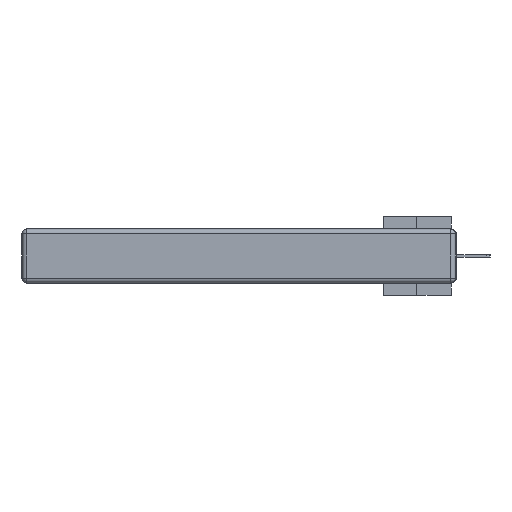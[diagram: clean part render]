
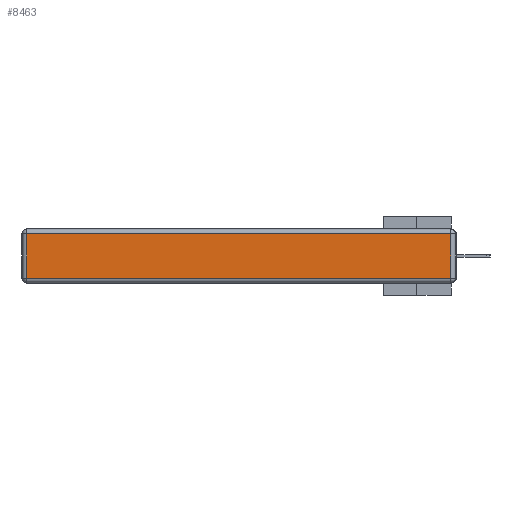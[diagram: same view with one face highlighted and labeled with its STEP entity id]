
A CAD part, left-side view. The second image highlights one B-rep face of the part: STEP entity #8463.
In plain terms, the highlighted planar face has unit normal (-1, 0, 0).
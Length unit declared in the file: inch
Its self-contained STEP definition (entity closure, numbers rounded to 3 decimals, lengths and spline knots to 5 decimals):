
#387 = VERTEX_POINT ( 'NONE', #8838 ) ;
#856 = VERTEX_POINT ( 'NONE', #28728 ) ;
#1134 = DIRECTION ( 'NONE',  ( 0., 0., -1. ) ) ;
#1557 = EDGE_CURVE ( 'NONE', #30566, #7993, #21441, .T. ) ;
#2081 = EDGE_CURVE ( 'NONE', #856, #387, #15373, .T. ) ;
#2544 = DIRECTION ( 'NONE',  ( -1., 0., 0. ) ) ;
#3279 = ORIENTED_EDGE ( 'NONE', *, *, #2081, .T. ) ;
#3412 = VECTOR ( 'NONE', #26601, 39.37008 ) ;
#4105 = EDGE_LOOP ( 'NONE', ( #13180, #20507, #6673, #3279 ) ) ;
#4881 = CARTESIAN_POINT ( 'NONE',  ( 0., 0., -0.343 ) ) ;
#6668 = VECTOR ( 'NONE', #13148, 39.37008 ) ;
#6673 = ORIENTED_EDGE ( 'NONE', *, *, #18201, .T. ) ;
#7993 = VERTEX_POINT ( 'NONE', #28312 ) ;
#8420 = CARTESIAN_POINT ( 'NONE',  ( 0., 2.72, -0.343 ) ) ;
#8463 = ADVANCED_FACE ( 'NONE', ( #26084 ), #23743, .T. ) ;
#8838 = CARTESIAN_POINT ( 'NONE',  ( 0., 2.72, -0.313 ) ) ;
#9593 = CARTESIAN_POINT ( 'NONE',  ( 0., 2.75, -0.03 ) ) ;
#11919 = DIRECTION ( 'NONE',  ( 0., 1., 0. ) ) ;
#11995 = DIRECTION ( 'NONE',  ( 0., 0., 1. ) ) ;
#13148 = DIRECTION ( 'NONE',  ( 0., -1., 0. ) ) ;
#13180 = ORIENTED_EDGE ( 'NONE', *, *, #23139, .T. ) ;
#14557 = AXIS2_PLACEMENT_3D ( 'NONE', #4881, #2544, #11995 ) ;
#15373 = LINE ( 'NONE', #8420, #22753 ) ;
#18201 = EDGE_CURVE ( 'NONE', #7993, #856, #23813, .T. ) ;
#18370 = CARTESIAN_POINT ( 'NONE',  ( 0., 0., -0.313 ) ) ;
#20266 = VECTOR ( 'NONE', #11919, 39.37008 ) ;
#20478 = CARTESIAN_POINT ( 'NONE',  ( 0., 0.03, -0.313 ) ) ;
#20507 = ORIENTED_EDGE ( 'NONE', *, *, #1557, .T. ) ;
#21441 = LINE ( 'NONE', #21593, #3412 ) ;
#21593 = CARTESIAN_POINT ( 'NONE',  ( 0., 0.03, -0.343 ) ) ;
#22753 = VECTOR ( 'NONE', #1134, 39.37008 ) ;
#23139 = EDGE_CURVE ( 'NONE', #387, #30566, #27885, .T. ) ;
#23743 = PLANE ( 'NONE',  #14557 ) ;
#23813 = LINE ( 'NONE', #9593, #20266 ) ;
#26084 = FACE_OUTER_BOUND ( 'NONE', #4105, .T. ) ;
#26601 = DIRECTION ( 'NONE',  ( 0., 0., 1. ) ) ;
#27885 = LINE ( 'NONE', #18370, #6668 ) ;
#28312 = CARTESIAN_POINT ( 'NONE',  ( 0., 0.03, -0.03 ) ) ;
#28728 = CARTESIAN_POINT ( 'NONE',  ( 0., 2.72, -0.03 ) ) ;
#30566 = VERTEX_POINT ( 'NONE', #20478 ) ;
